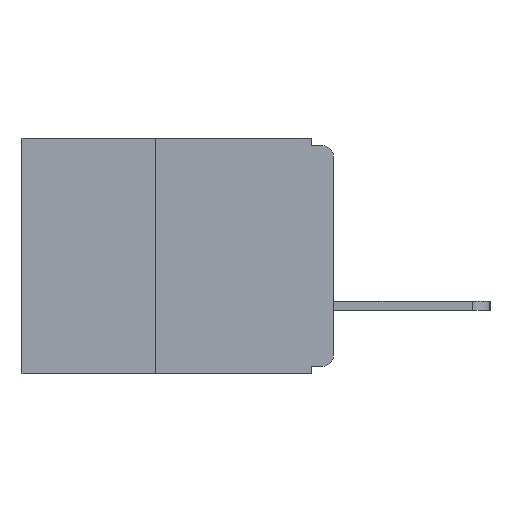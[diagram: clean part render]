
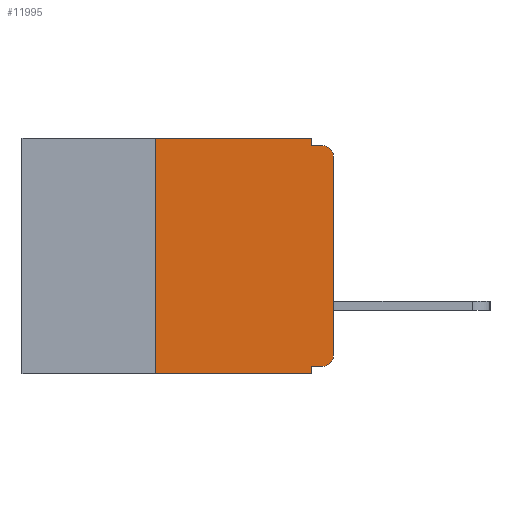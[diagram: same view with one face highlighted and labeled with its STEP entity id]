
A CAD part, left-side view. The second image highlights one B-rep face of the part: STEP entity #11995.
In plain terms, the highlighted planar face has unit normal (-1, 0, 0).
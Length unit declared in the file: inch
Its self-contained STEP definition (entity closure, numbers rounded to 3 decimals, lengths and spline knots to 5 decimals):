
#134 = EDGE_CURVE ( 'NONE', #7901, #16925, #9057, .T. ) ;
#259 = ORIENTED_EDGE ( 'NONE', *, *, #14188, .F. ) ;
#315 = ORIENTED_EDGE ( 'NONE', *, *, #15310, .T. ) ;
#416 = EDGE_CURVE ( 'NONE', #2037, #16925, #14071, .T. ) ;
#691 = EDGE_CURVE ( 'NONE', #5258, #8839, #9683, .T. ) ;
#912 = CARTESIAN_POINT ( 'NONE',  ( 0., 0., -0.025 ) ) ;
#916 = CARTESIAN_POINT ( 'NONE',  ( 0., 0.031, -0.01 ) ) ;
#1108 = ORIENTED_EDGE ( 'NONE', *, *, #13562, .F. ) ;
#1150 = ORIENTED_EDGE ( 'NONE', *, *, #691, .T. ) ;
#1466 = CARTESIAN_POINT ( 'NONE',  ( 0., 0.015, -0.305 ) ) ;
#1743 = FACE_OUTER_BOUND ( 'NONE', #7361, .T. ) ;
#2037 = VERTEX_POINT ( 'NONE', #916 ) ;
#2083 = ORIENTED_EDGE ( 'NONE', *, *, #12756, .T. ) ;
#2157 = DIRECTION ( 'NONE',  ( 0., -1., 0. ) ) ;
#2176 = CARTESIAN_POINT ( 'NONE',  ( 0., 0.031, -0.33 ) ) ;
#2433 = AXIS2_PLACEMENT_3D ( 'NONE', #5297, #7835, #5179 ) ;
#2448 = DIRECTION ( 'NONE',  ( 0., 0., -1. ) ) ;
#2614 = DIRECTION ( 'NONE',  ( 0., 1., 0. ) ) ;
#2667 = VECTOR ( 'NONE', #6955, 39.37008 ) ;
#2684 = LINE ( 'NONE', #10036, #15978 ) ;
#2702 = CARTESIAN_POINT ( 'NONE',  ( 0., 0.25, -0.33 ) ) ;
#2865 = ORIENTED_EDGE ( 'NONE', *, *, #134, .T. ) ;
#2969 = DIRECTION ( 'NONE',  ( -1., 0., 0. ) ) ;
#3098 = CARTESIAN_POINT ( 'NONE',  ( 0., 0., -0.01 ) ) ;
#3224 = DIRECTION ( 'NONE',  ( 1., 0., 0. ) ) ;
#3358 = EDGE_CURVE ( 'NONE', #5258, #11518, #12952, .T. ) ;
#3604 = VECTOR ( 'NONE', #2614, 39.37008 ) ;
#3620 = CARTESIAN_POINT ( 'NONE',  ( 0., 0.031, 0. ) ) ;
#3781 = CARTESIAN_POINT ( 'NONE',  ( 0., 0., 0. ) ) ;
#3910 = VECTOR ( 'NONE', #14903, 39.37008 ) ;
#4570 = CARTESIAN_POINT ( 'NONE',  ( 0., 0.437, 0. ) ) ;
#5179 = DIRECTION ( 'NONE',  ( 0., 0., -1. ) ) ;
#5258 = VERTEX_POINT ( 'NONE', #10162 ) ;
#5297 = CARTESIAN_POINT ( 'NONE',  ( 0., 0.015, -0.025 ) ) ;
#6372 = VERTEX_POINT ( 'NONE', #12649 ) ;
#6488 = CARTESIAN_POINT ( 'NONE',  ( 0., 0., -0.32 ) ) ;
#6955 = DIRECTION ( 'NONE',  ( 0., -1., 0. ) ) ;
#7219 = ORIENTED_EDGE ( 'NONE', *, *, #9944, .F. ) ;
#7228 = LINE ( 'NONE', #2176, #14549 ) ;
#7253 = DIRECTION ( 'NONE',  ( 0., 0., 1. ) ) ;
#7284 = LINE ( 'NONE', #4570, #13969 ) ;
#7361 = EDGE_LOOP ( 'NONE', ( #315, #2865, #17185, #259, #9750, #1108, #2083, #7219, #14761, #1150 ) ) ;
#7381 = LINE ( 'NONE', #9598, #3910 ) ;
#7427 = CARTESIAN_POINT ( 'NONE',  ( 0., 0.031, -0.33 ) ) ;
#7631 = VERTEX_POINT ( 'NONE', #3620 ) ;
#7754 = VERTEX_POINT ( 'NONE', #2702 ) ;
#7835 = DIRECTION ( 'NONE',  ( -1., 0., 0. ) ) ;
#7901 = VERTEX_POINT ( 'NONE', #912 ) ;
#8349 = CARTESIAN_POINT ( 'NONE',  ( 0., 0.437, 0. ) ) ;
#8839 = VERTEX_POINT ( 'NONE', #14475 ) ;
#8931 = AXIS2_PLACEMENT_3D ( 'NONE', #8349, #3224, #15171 ) ;
#9057 = CIRCLE ( 'NONE', #2433, 0.015 ) ;
#9450 = VECTOR ( 'NONE', #2448, 39.37008 ) ;
#9598 = CARTESIAN_POINT ( 'NONE',  ( 0., 0.25, -0.33 ) ) ;
#9683 = CIRCLE ( 'NONE', #16667, 0.015 ) ;
#9750 = ORIENTED_EDGE ( 'NONE', *, *, #16100, .F. ) ;
#9944 = EDGE_CURVE ( 'NONE', #11518, #15815, #7228, .T. ) ;
#10036 = CARTESIAN_POINT ( 'NONE',  ( 0., 0.437, -0.33 ) ) ;
#10162 = CARTESIAN_POINT ( 'NONE',  ( 0., 0.015, -0.32 ) ) ;
#10406 = CARTESIAN_POINT ( 'NONE',  ( 0., 0.031, 0. ) ) ;
#11373 = DIRECTION ( 'NONE',  ( 0., 0., -1. ) ) ;
#11518 = VERTEX_POINT ( 'NONE', #14798 ) ;
#11995 = ADVANCED_FACE ( 'NONE', ( #1743 ), #12401, .F. ) ;
#12313 = DIRECTION ( 'NONE',  ( 0., 0., -1. ) ) ;
#12401 = PLANE ( 'NONE',  #8931 ) ;
#12607 = CARTESIAN_POINT ( 'NONE',  ( 0., 0.015, -0.01 ) ) ;
#12649 = CARTESIAN_POINT ( 'NONE',  ( 0., 0.25, 0. ) ) ;
#12756 = EDGE_CURVE ( 'NONE', #7754, #15815, #2684, .T. ) ;
#12759 = VECTOR ( 'NONE', #7253, 39.37008 ) ;
#12952 = LINE ( 'NONE', #6488, #3604 ) ;
#13562 = EDGE_CURVE ( 'NONE', #7754, #6372, #7381, .T. ) ;
#13965 = DIRECTION ( 'NONE',  ( 0., -1., 0. ) ) ;
#13969 = VECTOR ( 'NONE', #13965, 39.37008 ) ;
#14004 = LINE ( 'NONE', #3781, #12759 ) ;
#14071 = LINE ( 'NONE', #3098, #2667 ) ;
#14188 = EDGE_CURVE ( 'NONE', #7631, #2037, #15079, .T. ) ;
#14475 = CARTESIAN_POINT ( 'NONE',  ( 0., 0., -0.305 ) ) ;
#14549 = VECTOR ( 'NONE', #11373, 39.37008 ) ;
#14761 = ORIENTED_EDGE ( 'NONE', *, *, #3358, .F. ) ;
#14798 = CARTESIAN_POINT ( 'NONE',  ( 0., 0.031, -0.32 ) ) ;
#14903 = DIRECTION ( 'NONE',  ( 0., 0., 1. ) ) ;
#15079 = LINE ( 'NONE', #10406, #9450 ) ;
#15171 = DIRECTION ( 'NONE',  ( 0., 0., -1. ) ) ;
#15310 = EDGE_CURVE ( 'NONE', #8839, #7901, #14004, .T. ) ;
#15815 = VERTEX_POINT ( 'NONE', #7427 ) ;
#15978 = VECTOR ( 'NONE', #2157, 39.37008 ) ;
#16100 = EDGE_CURVE ( 'NONE', #6372, #7631, #7284, .T. ) ;
#16667 = AXIS2_PLACEMENT_3D ( 'NONE', #1466, #2969, #12313 ) ;
#16925 = VERTEX_POINT ( 'NONE', #12607 ) ;
#17185 = ORIENTED_EDGE ( 'NONE', *, *, #416, .F. ) ;
